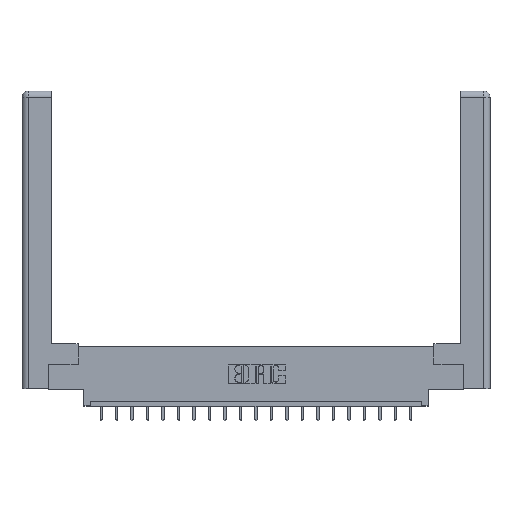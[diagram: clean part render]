
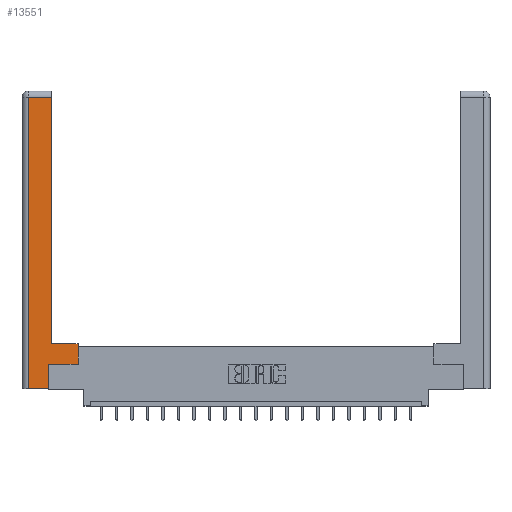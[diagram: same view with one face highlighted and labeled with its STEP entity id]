
A CAD part, top view. The second image highlights one B-rep face of the part: STEP entity #13551.
In plain terms, the highlighted planar face has unit normal (0, 0, 1).
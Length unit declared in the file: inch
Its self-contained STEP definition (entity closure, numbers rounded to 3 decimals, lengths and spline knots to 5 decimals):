
#200 = VERTEX_POINT ( 'NONE', #18581 ) ;
#402 = LINE ( 'NONE', #3911, #2206 ) ;
#433 = ORIENTED_EDGE ( 'NONE', *, *, #15140, .T. ) ;
#623 = LINE ( 'NONE', #20094, #6506 ) ;
#1104 = VECTOR ( 'NONE', #13330, 39.37008 ) ;
#1605 = ORIENTED_EDGE ( 'NONE', *, *, #5196, .T. ) ;
#2206 = VECTOR ( 'NONE', #10262, 39.37008 ) ;
#2830 = LINE ( 'NONE', #12434, #4863 ) ;
#2861 = DIRECTION ( 'NONE',  ( -1., 0., 0. ) ) ;
#3152 = EDGE_CURVE ( 'NONE', #7887, #3178, #5293, .T. ) ;
#3178 = VERTEX_POINT ( 'NONE', #11094 ) ;
#3648 = CARTESIAN_POINT ( 'NONE',  ( 0.295, 3., 0. ) ) ;
#3911 = CARTESIAN_POINT ( 'NONE',  ( 0.265, 0.245, 0. ) ) ;
#4215 = CARTESIAN_POINT ( 'NONE',  ( 0.295, 0.45, 0. ) ) ;
#4373 = CARTESIAN_POINT ( 'NONE',  ( 0.295, 2.94, 0. ) ) ;
#4520 = VECTOR ( 'NONE', #10567, 39.37008 ) ;
#4863 = VECTOR ( 'NONE', #10862, 39.37008 ) ;
#5049 = FACE_OUTER_BOUND ( 'NONE', #19051, .T. ) ;
#5196 = EDGE_CURVE ( 'NONE', #10666, #18148, #12561, .T. ) ;
#5197 = VECTOR ( 'NONE', #10470, 39.37008 ) ;
#5293 = LINE ( 'NONE', #11239, #21097 ) ;
#5792 = ORIENTED_EDGE ( 'NONE', *, *, #15581, .T. ) ;
#6034 = CARTESIAN_POINT ( 'NONE',  ( 0.265, 0.245, 0. ) ) ;
#6057 = EDGE_CURVE ( 'NONE', #200, #17012, #9783, .T. ) ;
#6506 = VECTOR ( 'NONE', #13850, 39.37008 ) ;
#7579 = DIRECTION ( 'NONE',  ( 0., 0., -1. ) ) ;
#7887 = VERTEX_POINT ( 'NONE', #8875 ) ;
#8149 = ORIENTED_EDGE ( 'NONE', *, *, #16300, .T. ) ;
#8684 = CARTESIAN_POINT ( 'NONE',  ( 0.0615, 2.94, 0. ) ) ;
#8745 = ORIENTED_EDGE ( 'NONE', *, *, #10293, .T. ) ;
#8875 = CARTESIAN_POINT ( 'NONE',  ( 0.565, 0.245, 0. ) ) ;
#9268 = CARTESIAN_POINT ( 'NONE',  ( 0.265, 0., 0. ) ) ;
#9371 = LINE ( 'NONE', #4215, #4520 ) ;
#9739 = VECTOR ( 'NONE', #18083, 39.37008 ) ;
#9783 = LINE ( 'NONE', #11734, #1104 ) ;
#10111 = CARTESIAN_POINT ( 'NONE',  ( 0.295, 0.45, 0. ) ) ;
#10262 = DIRECTION ( 'NONE',  ( 0., 1., 0. ) ) ;
#10293 = EDGE_CURVE ( 'NONE', #3178, #10666, #9371, .T. ) ;
#10470 = DIRECTION ( 'NONE',  ( 1., 0., 0. ) ) ;
#10567 = DIRECTION ( 'NONE',  ( -1., 0., 0. ) ) ;
#10666 = VERTEX_POINT ( 'NONE', #10111 ) ;
#10862 = DIRECTION ( 'NONE',  ( 0., -1., 0. ) ) ;
#11094 = CARTESIAN_POINT ( 'NONE',  ( 0.565, 0.45, 0. ) ) ;
#11239 = CARTESIAN_POINT ( 'NONE',  ( 0.565, 0.45, 0. ) ) ;
#11707 = ORIENTED_EDGE ( 'NONE', *, *, #6057, .T. ) ;
#11734 = CARTESIAN_POINT ( 'NONE',  ( 0.265, 0., 0. ) ) ;
#12132 = VERTEX_POINT ( 'NONE', #8684 ) ;
#12203 = EDGE_CURVE ( 'NONE', #12472, #7887, #13158, .T. ) ;
#12434 = CARTESIAN_POINT ( 'NONE',  ( 0.0615, 0., 0. ) ) ;
#12472 = VERTEX_POINT ( 'NONE', #6034 ) ;
#12507 = CARTESIAN_POINT ( 'NONE',  ( 0., 0., 0. ) ) ;
#12561 = LINE ( 'NONE', #3648, #9739 ) ;
#13158 = LINE ( 'NONE', #16964, #5197 ) ;
#13330 = DIRECTION ( 'NONE',  ( 1., 0., 0. ) ) ;
#13551 = ADVANCED_FACE ( 'NONE', ( #5049 ), #20751, .F. ) ;
#13850 = DIRECTION ( 'NONE',  ( -1., 0., 0. ) ) ;
#14336 = DIRECTION ( 'NONE',  ( 0., 1., 0. ) ) ;
#15140 = EDGE_CURVE ( 'NONE', #17012, #12472, #402, .T. ) ;
#15581 = EDGE_CURVE ( 'NONE', #18148, #12132, #623, .T. ) ;
#16300 = EDGE_CURVE ( 'NONE', #12132, #200, #2830, .T. ) ;
#16833 = AXIS2_PLACEMENT_3D ( 'NONE', #12507, #7579, #2861 ) ;
#16964 = CARTESIAN_POINT ( 'NONE',  ( 0.565, 0.245, 0. ) ) ;
#16994 = ORIENTED_EDGE ( 'NONE', *, *, #12203, .T. ) ;
#17012 = VERTEX_POINT ( 'NONE', #9268 ) ;
#18083 = DIRECTION ( 'NONE',  ( 0., 1., 0. ) ) ;
#18148 = VERTEX_POINT ( 'NONE', #4373 ) ;
#18581 = CARTESIAN_POINT ( 'NONE',  ( 0.0615, 0., 0. ) ) ;
#19051 = EDGE_LOOP ( 'NONE', ( #1605, #5792, #8149, #11707, #433, #16994, #20964, #8745 ) ) ;
#20094 = CARTESIAN_POINT ( 'NONE',  ( 0.0615, 2.94, 0. ) ) ;
#20751 = PLANE ( 'NONE',  #16833 ) ;
#20964 = ORIENTED_EDGE ( 'NONE', *, *, #3152, .T. ) ;
#21097 = VECTOR ( 'NONE', #14336, 39.37008 ) ;
